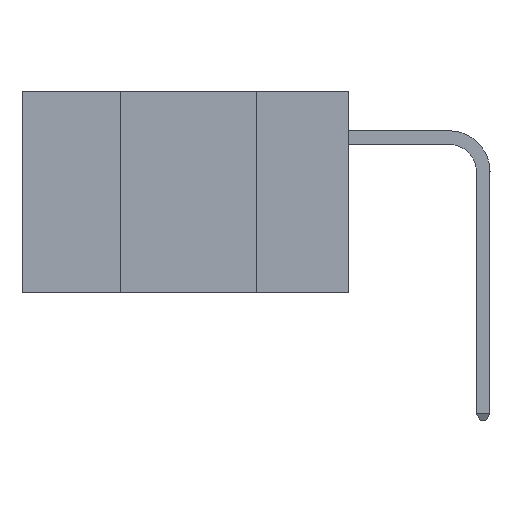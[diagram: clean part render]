
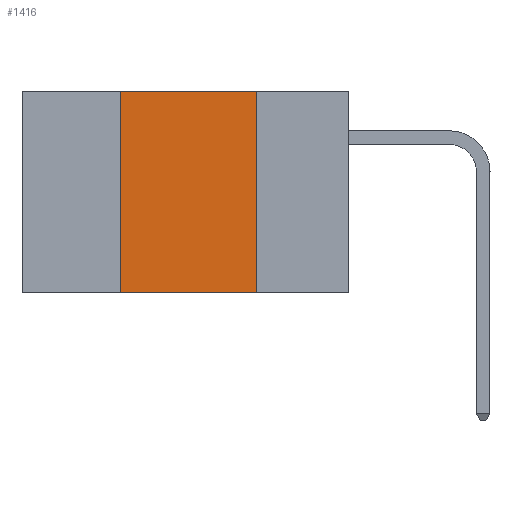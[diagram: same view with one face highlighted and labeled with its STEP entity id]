
A CAD part, left-side view. The second image highlights one B-rep face of the part: STEP entity #1416.
In plain terms, the highlighted planar face has unit normal (-1, 0, 0).
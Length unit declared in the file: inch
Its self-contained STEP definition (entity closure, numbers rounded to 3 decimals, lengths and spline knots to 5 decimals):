
#232 = DIRECTION ( 'NONE',  ( 0., -1., 0. ) ) ;
#395 = EDGE_CURVE ( 'NONE', #17005, #16880, #6856, .T. ) ;
#1046 = CARTESIAN_POINT ( 'NONE',  ( 0., 0.6, 0. ) ) ;
#1093 = VERTEX_POINT ( 'NONE', #15086 ) ;
#1416 = ADVANCED_FACE ( 'NONE', ( #5246 ), #19433, .F. ) ;
#3126 = CARTESIAN_POINT ( 'NONE',  ( 0., 0.6, 0. ) ) ;
#3399 = LINE ( 'NONE', #25872, #10705 ) ;
#4490 = DIRECTION ( 'NONE',  ( 0., 0., 1. ) ) ;
#5168 = CARTESIAN_POINT ( 'NONE',  ( 0., 0.6, -0.37 ) ) ;
#5216 = EDGE_CURVE ( 'NONE', #20244, #1093, #23784, .T. ) ;
#5246 = FACE_OUTER_BOUND ( 'NONE', #11329, .T. ) ;
#5847 = AXIS2_PLACEMENT_3D ( 'NONE', #1046, #12639, #14445 ) ;
#6856 = LINE ( 'NONE', #5168, #8874 ) ;
#8535 = ORIENTED_EDGE ( 'NONE', *, *, #20809, .F. ) ;
#8874 = VECTOR ( 'NONE', #232, 39.37008 ) ;
#10383 = VECTOR ( 'NONE', #12324, 39.37008 ) ;
#10705 = VECTOR ( 'NONE', #21652, 39.37008 ) ;
#11329 = EDGE_LOOP ( 'NONE', ( #23196, #27503, #8535, #21772 ) ) ;
#12324 = DIRECTION ( 'NONE',  ( 0., -1., 0. ) ) ;
#12639 = DIRECTION ( 'NONE',  ( 1., 0., 0. ) ) ;
#13902 = VECTOR ( 'NONE', #4490, 39.37008 ) ;
#14445 = DIRECTION ( 'NONE',  ( 0., 0., -1. ) ) ;
#15086 = CARTESIAN_POINT ( 'NONE',  ( 0., 0.17, 0. ) ) ;
#16393 = CARTESIAN_POINT ( 'NONE',  ( 0., 0.42, 0. ) ) ;
#16880 = VERTEX_POINT ( 'NONE', #18548 ) ;
#17005 = VERTEX_POINT ( 'NONE', #19134 ) ;
#18548 = CARTESIAN_POINT ( 'NONE',  ( 0., 0.17, -0.37 ) ) ;
#19134 = CARTESIAN_POINT ( 'NONE',  ( 0., 0.42, -0.37 ) ) ;
#19433 = PLANE ( 'NONE',  #5847 ) ;
#20244 = VERTEX_POINT ( 'NONE', #21926 ) ;
#20809 = EDGE_CURVE ( 'NONE', #17005, #20244, #23194, .T. ) ;
#21652 = DIRECTION ( 'NONE',  ( 0., 0., -1. ) ) ;
#21772 = ORIENTED_EDGE ( 'NONE', *, *, #395, .T. ) ;
#21926 = CARTESIAN_POINT ( 'NONE',  ( 0., 0.42, 0. ) ) ;
#23194 = LINE ( 'NONE', #16393, #13902 ) ;
#23196 = ORIENTED_EDGE ( 'NONE', *, *, #26074, .F. ) ;
#23784 = LINE ( 'NONE', #3126, #10383 ) ;
#25872 = CARTESIAN_POINT ( 'NONE',  ( 0., 0.17, 0. ) ) ;
#26074 = EDGE_CURVE ( 'NONE', #1093, #16880, #3399, .T. ) ;
#27503 = ORIENTED_EDGE ( 'NONE', *, *, #5216, .F. ) ;
